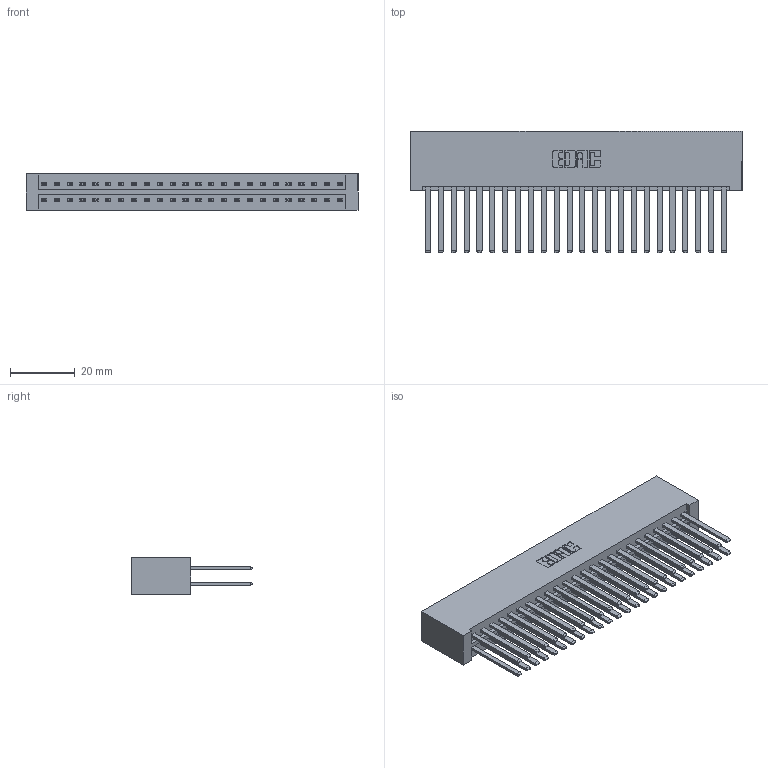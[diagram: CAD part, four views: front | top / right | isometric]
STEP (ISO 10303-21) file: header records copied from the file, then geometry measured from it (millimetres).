
FILE_DESCRIPTION (( 'STEP AP203' ), '1' );
FILE_NAME ('336-048-541-801.STEP', '2020-08-08T00:00:55', ( '' ), ( '' ), 'SwSTEP 2.0', 'SolidWorks 2020', '' );
FILE_SCHEMA (( 'CONFIG_CONTROL_DESIGN' ));
Length unit declared in the file: inch
Products named in the file (3): 336-290-001_336-290-541; 336-048-541-801; 336 Part_Lugless
Assembly tree (49 placements, depth 2):
  336-048-541-801
    336 Part_Lugless
    336-290-001_336-290-541  x48
Bounding box: 102.21 x 37.34 x 11.1 mm (x, y, z)
Volume: 16880.8 mm3; surface area: 21417.3 mm2
Topology: 49 solids, 49 shells, 2122 faces, 6383 edges, 4222 vertices
Faces by surface type: plane 1314, cylinder 808
Entity records: 20378 total; most frequent: CARTESIAN_POINT 3529, ORIENTED_EDGE 3366, DIRECTION 2931, EDGE_CURVE 1683, LINE 1559, VECTOR 1559, VERTEX_POINT 1120, AXIS2_PLACEMENT_3D 686
